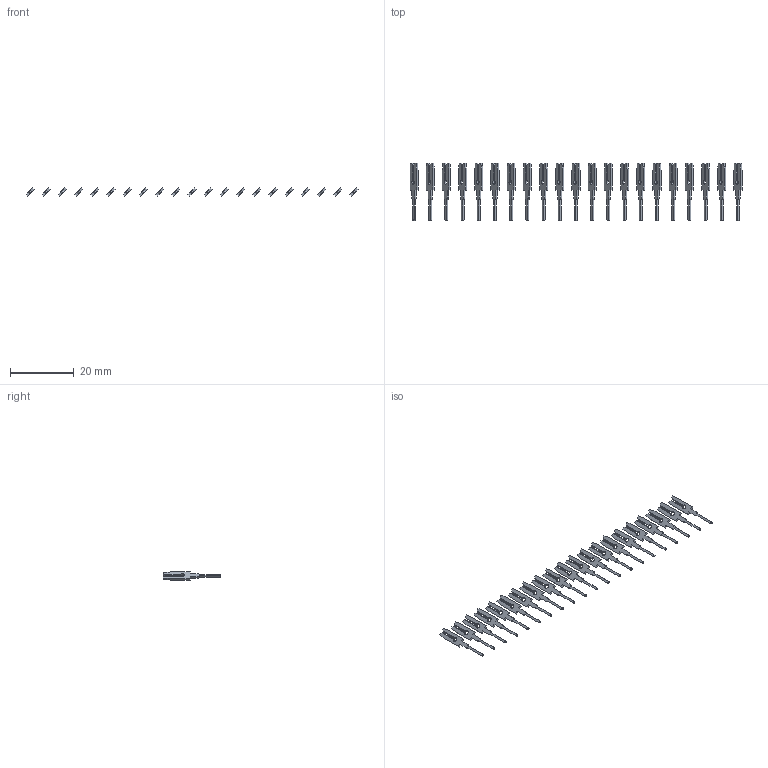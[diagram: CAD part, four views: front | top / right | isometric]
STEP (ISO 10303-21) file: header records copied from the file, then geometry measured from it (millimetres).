
FILE_DESCRIPTION (( 'STEP AP203' ), '1' );
FILE_NAME ('106-021-251-200.STEP', '2020-04-16T19:15:17', ( '' ), ( '' ), 'SwSTEP 2.0', 'SolidWorks 2016', '' );
FILE_SCHEMA (( 'CONFIG_CONTROL_DESIGN' ));
Length unit declared in the file: inch
Products named in the file (2): 106-021-251-200; 100-290-001_100-290-251
Assembly tree (21 placements, depth 2):
  106-021-251-200
    100-290-001_100-290-251  x21
Bounding box: 104.13 x 17.91 x 2.53 mm (x, y, z)
Volume: 384 mm3; surface area: 1887.2 mm2
Topology: 21 solids, 21 shells, 588 faces, 1638 edges, 1092 vertices
Faces by surface type: plane 462, cylinder 126
Entity records: 1734 total; most frequent: CARTESIAN_POINT 194, DIRECTION 190, ORIENTED_EDGE 156, EDGE_CURVE 78, AXIS2_PLACEMENT_3D 64, LINE 62, VECTOR 62, COORDINATED_UNIVERSAL_TIME_OFFSET 52
